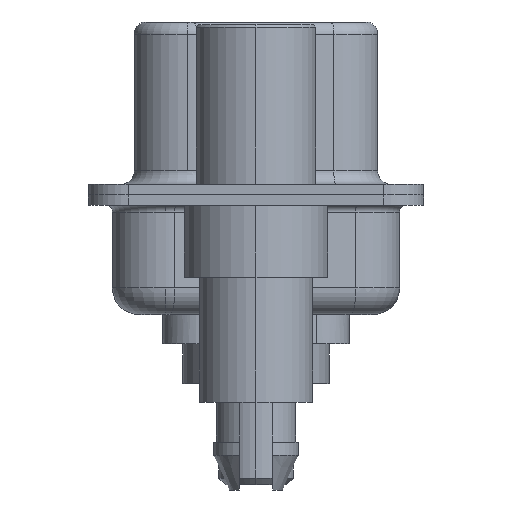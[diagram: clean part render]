
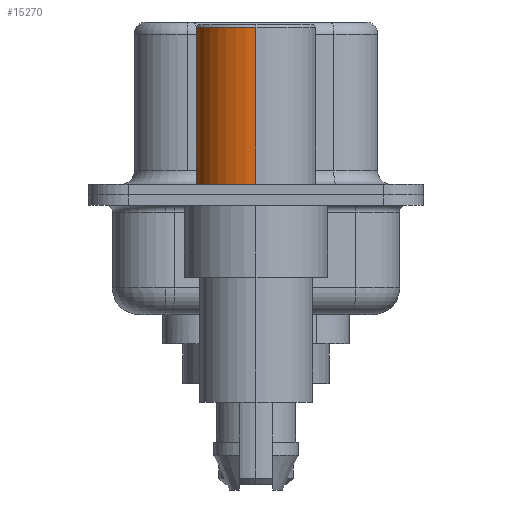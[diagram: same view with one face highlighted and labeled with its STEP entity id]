
A CAD part, left-side view. The second image highlights one B-rep face of the part: STEP entity #15270.
In plain terms, the highlighted cylindrical face has radius 2.25 mm (diameter 4.5 mm), a partial arc.
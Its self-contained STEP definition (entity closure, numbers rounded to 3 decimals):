
#346 = CYLINDRICAL_SURFACE ( 'NONE', #1471, 2.25 ) ;
#357 = EDGE_CURVE ( 'NONE', #16385, #11603, #16203, .T. ) ;
#956 = CARTESIAN_POINT ( 'NONE',  ( 2.25, 0., 6.3 ) ) ;
#1201 = DIRECTION ( 'NONE',  ( 0., 0., 1. ) ) ;
#1471 = AXIS2_PLACEMENT_3D ( 'NONE', #3199, #4546, #12859 ) ;
#1494 = VECTOR ( 'NONE', #1201, 1000. ) ;
#1533 = CIRCLE ( 'NONE', #17327, 2.25 ) ;
#1626 = CARTESIAN_POINT ( 'NONE',  ( -2.25, 0., 6.3 ) ) ;
#1943 = EDGE_CURVE ( 'NONE', #11603, #9436, #13321, .T. ) ;
#3026 = EDGE_CURVE ( 'NONE', #5465, #9436, #4617, .T. ) ;
#3164 = DIRECTION ( 'NONE',  ( 0., 0., 1. ) ) ;
#3199 = CARTESIAN_POINT ( 'NONE',  ( 0., 0., 0.581 ) ) ;
#3463 = CARTESIAN_POINT ( 'NONE',  ( -2.25, 0., 0.581 ) ) ;
#3767 = DIRECTION ( 'NONE',  ( 0., 0., 1. ) ) ;
#4546 = DIRECTION ( 'NONE',  ( 0., 0., 1. ) ) ;
#4617 = LINE ( 'NONE', #3463, #11481 ) ;
#4966 = DIRECTION ( 'NONE',  ( 1., 0., 0. ) ) ;
#5095 = DIRECTION ( 'NONE',  ( 0., 0., 1. ) ) ;
#5152 = CARTESIAN_POINT ( 'NONE',  ( 0., 0., 6.3 ) ) ;
#5345 = EDGE_CURVE ( 'NONE', #16385, #5465, #1533, .T. ) ;
#5465 = VERTEX_POINT ( 'NONE', #7993 ) ;
#7667 = FACE_OUTER_BOUND ( 'NONE', #12304, .T. ) ;
#7993 = CARTESIAN_POINT ( 'NONE',  ( -2.25, 0., 0.4 ) ) ;
#9381 = CARTESIAN_POINT ( 'NONE',  ( 0., 0., 0.4 ) ) ;
#9436 = VERTEX_POINT ( 'NONE', #1626 ) ;
#11481 = VECTOR ( 'NONE', #3164, 1000. ) ;
#11603 = VERTEX_POINT ( 'NONE', #956 ) ;
#12304 = EDGE_LOOP ( 'NONE', ( #17305, #13196, #15009, #13531 ) ) ;
#12859 = DIRECTION ( 'NONE',  ( 1., 0., 0. ) ) ;
#13196 = ORIENTED_EDGE ( 'NONE', *, *, #3026, .T. ) ;
#13321 = CIRCLE ( 'NONE', #13388, 2.25 ) ;
#13388 = AXIS2_PLACEMENT_3D ( 'NONE', #5152, #5095, #4966 ) ;
#13531 = ORIENTED_EDGE ( 'NONE', *, *, #357, .F. ) ;
#14192 = CARTESIAN_POINT ( 'NONE',  ( 2.25, 0., 0.581 ) ) ;
#15009 = ORIENTED_EDGE ( 'NONE', *, *, #1943, .F. ) ;
#15077 = CARTESIAN_POINT ( 'NONE',  ( 2.25, 0., 0.4 ) ) ;
#15270 = ADVANCED_FACE ( 'NONE', ( #7667 ), #346, .T. ) ;
#16203 = LINE ( 'NONE', #14192, #1494 ) ;
#16385 = VERTEX_POINT ( 'NONE', #15077 ) ;
#17305 = ORIENTED_EDGE ( 'NONE', *, *, #5345, .T. ) ;
#17327 = AXIS2_PLACEMENT_3D ( 'NONE', #9381, #3767, #17392 ) ;
#17392 = DIRECTION ( 'NONE',  ( 1., 0., 0. ) ) ;
